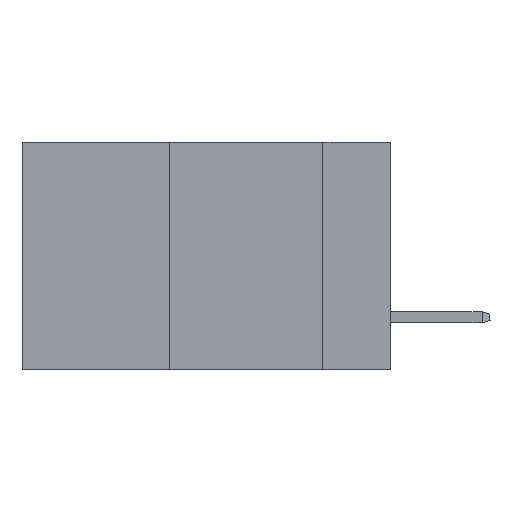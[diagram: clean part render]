
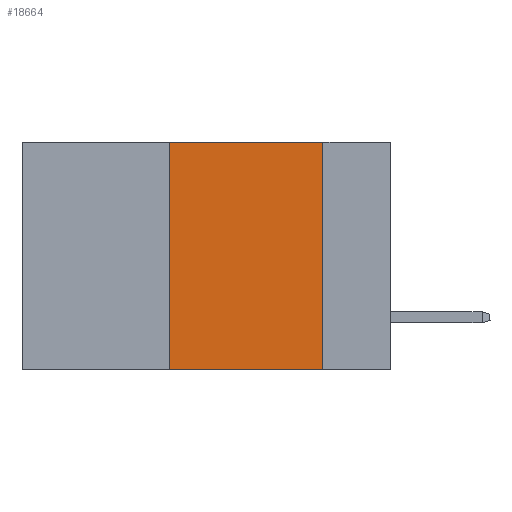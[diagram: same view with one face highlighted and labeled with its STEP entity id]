
A CAD part, left-side view. The second image highlights one B-rep face of the part: STEP entity #18664.
In plain terms, the highlighted planar face has unit normal (-1, 0, 0).
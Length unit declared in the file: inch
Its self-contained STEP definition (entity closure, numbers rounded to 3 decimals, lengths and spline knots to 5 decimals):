
#1189 = LINE ( 'NONE', #8259, #14494 ) ;
#1493 = VERTEX_POINT ( 'NONE', #12706 ) ;
#1702 = VERTEX_POINT ( 'NONE', #9322 ) ;
#1843 = ORIENTED_EDGE ( 'NONE', *, *, #7372, .F. ) ;
#2586 = DIRECTION ( 'NONE',  ( 0., -1., 0. ) ) ;
#2730 = LINE ( 'NONE', #4807, #8113 ) ;
#2948 = VERTEX_POINT ( 'NONE', #22130 ) ;
#3902 = EDGE_CURVE ( 'NONE', #1702, #1493, #22042, .T. ) ;
#4807 = CARTESIAN_POINT ( 'NONE',  ( 0., 0.36, 0. ) ) ;
#6097 = CARTESIAN_POINT ( 'NONE',  ( 0., 0.6, -0.37 ) ) ;
#6769 = DIRECTION ( 'NONE',  ( 0., 0., 1. ) ) ;
#7372 = EDGE_CURVE ( 'NONE', #1702, #10780, #2730, .T. ) ;
#7576 = LINE ( 'NONE', #18403, #19204 ) ;
#7846 = EDGE_CURVE ( 'NONE', #2948, #1493, #1189, .T. ) ;
#8113 = VECTOR ( 'NONE', #6769, 39.37008 ) ;
#8259 = CARTESIAN_POINT ( 'NONE',  ( 0., 0.11, 0. ) ) ;
#8577 = CARTESIAN_POINT ( 'NONE',  ( 0., 0.36, 0. ) ) ;
#9296 = DIRECTION ( 'NONE',  ( 0., 0., -1. ) ) ;
#9322 = CARTESIAN_POINT ( 'NONE',  ( 0., 0.36, -0.37 ) ) ;
#10341 = AXIS2_PLACEMENT_3D ( 'NONE', #20018, #18626, #9296 ) ;
#10780 = VERTEX_POINT ( 'NONE', #8577 ) ;
#11623 = PLANE ( 'NONE',  #10341 ) ;
#12706 = CARTESIAN_POINT ( 'NONE',  ( 0., 0.11, -0.37 ) ) ;
#14494 = VECTOR ( 'NONE', #22463, 39.37008 ) ;
#14541 = EDGE_CURVE ( 'NONE', #10780, #2948, #7576, .T. ) ;
#15083 = ORIENTED_EDGE ( 'NONE', *, *, #14541, .F. ) ;
#16865 = FACE_OUTER_BOUND ( 'NONE', #21762, .T. ) ;
#18403 = CARTESIAN_POINT ( 'NONE',  ( 0., 0.6, 0. ) ) ;
#18626 = DIRECTION ( 'NONE',  ( 1., 0., 0. ) ) ;
#18664 = ADVANCED_FACE ( 'NONE', ( #16865 ), #11623, .F. ) ;
#19204 = VECTOR ( 'NONE', #2586, 39.37008 ) ;
#20018 = CARTESIAN_POINT ( 'NONE',  ( 0., 0.6, 0. ) ) ;
#20038 = ORIENTED_EDGE ( 'NONE', *, *, #3902, .T. ) ;
#21532 = VECTOR ( 'NONE', #22285, 39.37008 ) ;
#21762 = EDGE_LOOP ( 'NONE', ( #22538, #15083, #1843, #20038 ) ) ;
#22042 = LINE ( 'NONE', #6097, #21532 ) ;
#22130 = CARTESIAN_POINT ( 'NONE',  ( 0., 0.11, 0. ) ) ;
#22285 = DIRECTION ( 'NONE',  ( 0., -1., 0. ) ) ;
#22463 = DIRECTION ( 'NONE',  ( 0., 0., -1. ) ) ;
#22538 = ORIENTED_EDGE ( 'NONE', *, *, #7846, .F. ) ;
